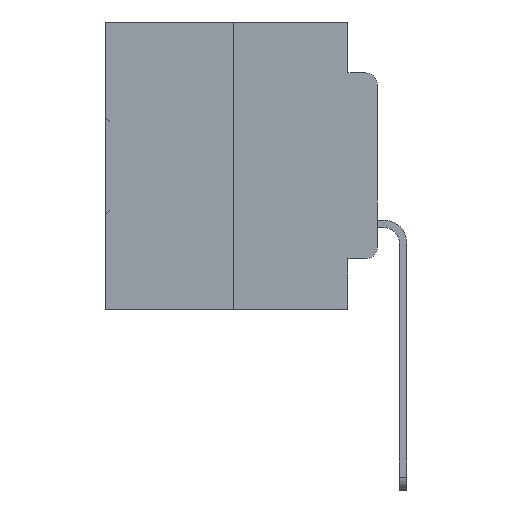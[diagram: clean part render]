
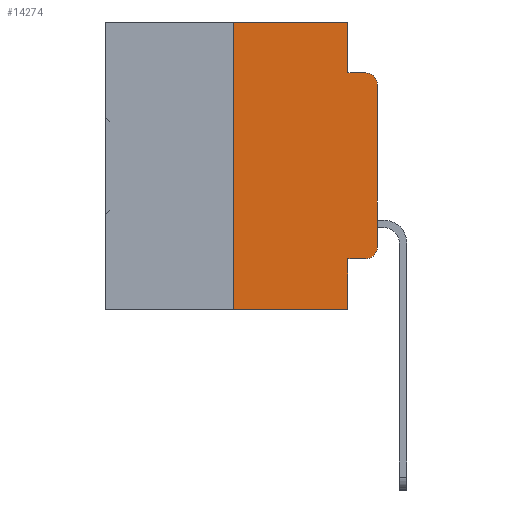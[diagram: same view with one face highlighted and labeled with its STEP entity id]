
A CAD part, left-side view. The second image highlights one B-rep face of the part: STEP entity #14274.
In plain terms, the highlighted planar face has unit normal (-1, 0, 0).
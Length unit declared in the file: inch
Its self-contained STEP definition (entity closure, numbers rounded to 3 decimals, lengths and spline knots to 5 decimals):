
#142 = VECTOR ( 'NONE', #16899, 39.37008 ) ;
#364 = CIRCLE ( 'NONE', #29703, 0.02 ) ;
#534 = VERTEX_POINT ( 'NONE', #10517 ) ;
#1053 = CARTESIAN_POINT ( 'NONE',  ( 0., 0.051, 0. ) ) ;
#1667 = LINE ( 'NONE', #27170, #21779 ) ;
#1782 = CARTESIAN_POINT ( 'NONE',  ( 0., 0., -0.1085 ) ) ;
#2036 = AXIS2_PLACEMENT_3D ( 'NONE', #15708, #33639, #18348 ) ;
#2920 = AXIS2_PLACEMENT_3D ( 'NONE', #17648, #20223, #4526 ) ;
#3256 = EDGE_LOOP ( 'NONE', ( #32588, #26992, #15384, #5753, #29573, #27169, #31221, #9655, #18650, #15371 ) ) ;
#3320 = VECTOR ( 'NONE', #16887, 39.37008 ) ;
#3563 = CARTESIAN_POINT ( 'NONE',  ( 0., 0., -0.3915 ) ) ;
#3670 = CARTESIAN_POINT ( 'NONE',  ( 0., 0.051, -0.0885 ) ) ;
#3823 = DIRECTION ( 'NONE',  ( 0., 0., -1. ) ) ;
#4057 = VERTEX_POINT ( 'NONE', #17888 ) ;
#4526 = DIRECTION ( 'NONE',  ( 0., 0., -1. ) ) ;
#4818 = EDGE_CURVE ( 'NONE', #5370, #15984, #18724, .T. ) ;
#5370 = VERTEX_POINT ( 'NONE', #28165 ) ;
#5753 = ORIENTED_EDGE ( 'NONE', *, *, #20626, .F. ) ;
#7284 = LINE ( 'NONE', #3670, #142 ) ;
#7346 = VERTEX_POINT ( 'NONE', #10104 ) ;
#7716 = EDGE_CURVE ( 'NONE', #15984, #17998, #1667, .T. ) ;
#8228 = CARTESIAN_POINT ( 'NONE',  ( 0., 0.02, -0.1085 ) ) ;
#8280 = VECTOR ( 'NONE', #3823, 39.37008 ) ;
#8387 = EDGE_CURVE ( 'NONE', #26216, #5370, #12317, .T. ) ;
#9373 = DIRECTION ( 'NONE',  ( 0., -1., 0. ) ) ;
#9655 = ORIENTED_EDGE ( 'NONE', *, *, #15399, .F. ) ;
#10087 = VECTOR ( 'NONE', #25411, 39.37008 ) ;
#10104 = CARTESIAN_POINT ( 'NONE',  ( 0., 0.051, -0.5 ) ) ;
#10517 = CARTESIAN_POINT ( 'NONE',  ( 0., 0.25, 0. ) ) ;
#10898 = DIRECTION ( 'NONE',  ( 0., 0., -1. ) ) ;
#12070 = CARTESIAN_POINT ( 'NONE',  ( 0., 0.25, -0.5 ) ) ;
#12317 = LINE ( 'NONE', #17137, #18482 ) ;
#12421 = VERTEX_POINT ( 'NONE', #12070 ) ;
#12996 = CARTESIAN_POINT ( 'NONE',  ( 0., 0.051, -0.0885 ) ) ;
#13122 = VERTEX_POINT ( 'NONE', #12996 ) ;
#14274 = ADVANCED_FACE ( 'NONE', ( #22205 ), #30388, .F. ) ;
#14300 = VECTOR ( 'NONE', #26246, 39.37008 ) ;
#14416 = LINE ( 'NONE', #22090, #8280 ) ;
#14693 = VERTEX_POINT ( 'NONE', #24543 ) ;
#15107 = LINE ( 'NONE', #15909, #14300 ) ;
#15371 = ORIENTED_EDGE ( 'NONE', *, *, #4818, .T. ) ;
#15384 = ORIENTED_EDGE ( 'NONE', *, *, #30899, .F. ) ;
#15399 = EDGE_CURVE ( 'NONE', #26216, #7346, #17310, .T. ) ;
#15708 = CARTESIAN_POINT ( 'NONE',  ( 0., 0.02, -0.3915 ) ) ;
#15909 = CARTESIAN_POINT ( 'NONE',  ( 0., 0.473, -0.5 ) ) ;
#15984 = VERTEX_POINT ( 'NONE', #3563 ) ;
#16887 = DIRECTION ( 'NONE',  ( 0., 0., -1. ) ) ;
#16899 = DIRECTION ( 'NONE',  ( 0., -1., 0. ) ) ;
#17063 = EDGE_CURVE ( 'NONE', #12421, #7346, #15107, .T. ) ;
#17137 = CARTESIAN_POINT ( 'NONE',  ( 0., 0.051, -0.4115 ) ) ;
#17310 = LINE ( 'NONE', #1053, #3320 ) ;
#17648 = CARTESIAN_POINT ( 'NONE',  ( 0., 0.473, 0. ) ) ;
#17888 = CARTESIAN_POINT ( 'NONE',  ( 0., 0.051, 0. ) ) ;
#17998 = VERTEX_POINT ( 'NONE', #1782 ) ;
#18348 = DIRECTION ( 'NONE',  ( 0., 0., -1. ) ) ;
#18482 = VECTOR ( 'NONE', #9373, 39.37008 ) ;
#18650 = ORIENTED_EDGE ( 'NONE', *, *, #8387, .T. ) ;
#18724 = CIRCLE ( 'NONE', #2036, 0.02 ) ;
#18919 = EDGE_CURVE ( 'NONE', #12421, #534, #24659, .T. ) ;
#20223 = DIRECTION ( 'NONE',  ( 1., 0., 0. ) ) ;
#20626 = EDGE_CURVE ( 'NONE', #4057, #13122, #14416, .T. ) ;
#21779 = VECTOR ( 'NONE', #32188, 39.37008 ) ;
#21793 = VECTOR ( 'NONE', #22680, 39.37008 ) ;
#22090 = CARTESIAN_POINT ( 'NONE',  ( 0., 0.051, 0. ) ) ;
#22205 = FACE_OUTER_BOUND ( 'NONE', #3256, .T. ) ;
#22584 = LINE ( 'NONE', #27726, #21793 ) ;
#22680 = DIRECTION ( 'NONE',  ( 0., -1., 0. ) ) ;
#24543 = CARTESIAN_POINT ( 'NONE',  ( 0., 0.02, -0.0885 ) ) ;
#24659 = LINE ( 'NONE', #33006, #10087 ) ;
#25411 = DIRECTION ( 'NONE',  ( 0., 0., 1. ) ) ;
#26216 = VERTEX_POINT ( 'NONE', #26362 ) ;
#26246 = DIRECTION ( 'NONE',  ( 0., -1., 0. ) ) ;
#26353 = DIRECTION ( 'NONE',  ( -1., 0., 0. ) ) ;
#26362 = CARTESIAN_POINT ( 'NONE',  ( 0., 0.051, -0.4115 ) ) ;
#26992 = ORIENTED_EDGE ( 'NONE', *, *, #32607, .T. ) ;
#27169 = ORIENTED_EDGE ( 'NONE', *, *, #18919, .F. ) ;
#27170 = CARTESIAN_POINT ( 'NONE',  ( 0., 0., 0. ) ) ;
#27726 = CARTESIAN_POINT ( 'NONE',  ( 0., 0.473, 0. ) ) ;
#28165 = CARTESIAN_POINT ( 'NONE',  ( 0., 0.02, -0.4115 ) ) ;
#29573 = ORIENTED_EDGE ( 'NONE', *, *, #32362, .F. ) ;
#29703 = AXIS2_PLACEMENT_3D ( 'NONE', #8228, #26353, #10898 ) ;
#30388 = PLANE ( 'NONE',  #2920 ) ;
#30899 = EDGE_CURVE ( 'NONE', #13122, #14693, #7284, .T. ) ;
#31221 = ORIENTED_EDGE ( 'NONE', *, *, #17063, .T. ) ;
#32188 = DIRECTION ( 'NONE',  ( 0., 0., 1. ) ) ;
#32362 = EDGE_CURVE ( 'NONE', #534, #4057, #22584, .T. ) ;
#32588 = ORIENTED_EDGE ( 'NONE', *, *, #7716, .T. ) ;
#32607 = EDGE_CURVE ( 'NONE', #17998, #14693, #364, .T. ) ;
#33006 = CARTESIAN_POINT ( 'NONE',  ( 0., 0.25, 0. ) ) ;
#33639 = DIRECTION ( 'NONE',  ( -1., 0., 0. ) ) ;
